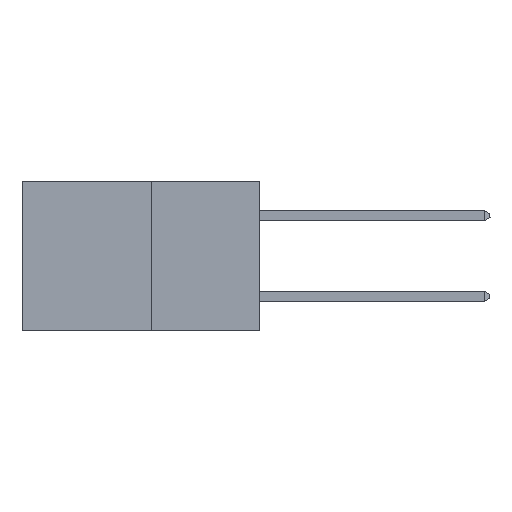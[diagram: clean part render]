
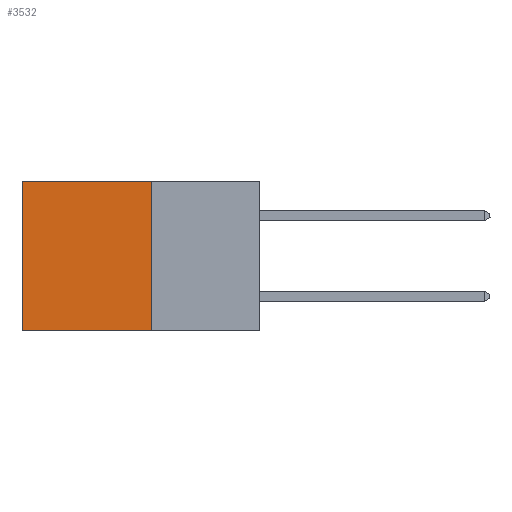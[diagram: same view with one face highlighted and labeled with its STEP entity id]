
A CAD part, left-side view. The second image highlights one B-rep face of the part: STEP entity #3532.
In plain terms, the highlighted planar face has unit normal (-1, 0, 0).
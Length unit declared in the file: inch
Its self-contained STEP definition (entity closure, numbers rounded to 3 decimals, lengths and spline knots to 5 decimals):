
#3 = DIRECTION ( 'NONE',  ( 0., 1., 0. ) ) ;
#212 = CARTESIAN_POINT ( 'NONE',  ( 0.277, 0.59, 0. ) ) ;
#484 = ORIENTED_EDGE ( 'NONE', *, *, #8022, .T. ) ;
#1516 = CARTESIAN_POINT ( 'NONE',  ( 0.277, 0.27, -0.37 ) ) ;
#1908 = CARTESIAN_POINT ( 'NONE',  ( 0.277, 0.59, -0.37 ) ) ;
#2278 = CARTESIAN_POINT ( 'NONE',  ( 0.277, 0.27, -0.37 ) ) ;
#2357 = DIRECTION ( 'NONE',  ( 1., 0., 0. ) ) ;
#2389 = DIRECTION ( 'NONE',  ( 0., 0., -1. ) ) ;
#2446 = EDGE_CURVE ( 'NONE', #5844, #5628, #2755, .T. ) ;
#2460 = AXIS2_PLACEMENT_3D ( 'NONE', #2278, #2357, #2389 ) ;
#2755 = LINE ( 'NONE', #9938, #9288 ) ;
#3532 = ADVANCED_FACE ( 'NONE', ( #8053 ), #4697, .F. ) ;
#3622 = LINE ( 'NONE', #16067, #13532 ) ;
#4187 = ORIENTED_EDGE ( 'NONE', *, *, #13033, .F. ) ;
#4394 = CARTESIAN_POINT ( 'NONE',  ( 0.277, 0.27, 0. ) ) ;
#4575 = ORIENTED_EDGE ( 'NONE', *, *, #14024, .F. ) ;
#4697 = PLANE ( 'NONE',  #2460 ) ;
#4932 = LINE ( 'NONE', #5967, #14796 ) ;
#5628 = VERTEX_POINT ( 'NONE', #1908 ) ;
#5844 = VERTEX_POINT ( 'NONE', #212 ) ;
#5967 = CARTESIAN_POINT ( 'NONE',  ( 0.277, 0.27, 0. ) ) ;
#6648 = VECTOR ( 'NONE', #3, 39.37008 ) ;
#6717 = EDGE_LOOP ( 'NONE', ( #7256, #4575, #4187, #484 ) ) ;
#7256 = ORIENTED_EDGE ( 'NONE', *, *, #2446, .T. ) ;
#8022 = EDGE_CURVE ( 'NONE', #16418, #5844, #4932, .T. ) ;
#8053 = FACE_OUTER_BOUND ( 'NONE', #6717, .T. ) ;
#8887 = LINE ( 'NONE', #13043, #6648 ) ;
#9288 = VECTOR ( 'NONE', #15565, 39.37008 ) ;
#9938 = CARTESIAN_POINT ( 'NONE',  ( 0.277, 0.59, -0.37 ) ) ;
#13033 = EDGE_CURVE ( 'NONE', #16418, #13436, #3622, .T. ) ;
#13043 = CARTESIAN_POINT ( 'NONE',  ( 0.277, 0.27, -0.37 ) ) ;
#13436 = VERTEX_POINT ( 'NONE', #1516 ) ;
#13532 = VECTOR ( 'NONE', #13598, 39.37008 ) ;
#13598 = DIRECTION ( 'NONE',  ( 0., 0., -1. ) ) ;
#14024 = EDGE_CURVE ( 'NONE', #13436, #5628, #8887, .T. ) ;
#14796 = VECTOR ( 'NONE', #14981, 39.37008 ) ;
#14981 = DIRECTION ( 'NONE',  ( 0., 1., 0. ) ) ;
#15565 = DIRECTION ( 'NONE',  ( 0., 0., -1. ) ) ;
#16067 = CARTESIAN_POINT ( 'NONE',  ( 0.277, 0.27, -0.37 ) ) ;
#16418 = VERTEX_POINT ( 'NONE', #4394 ) ;
